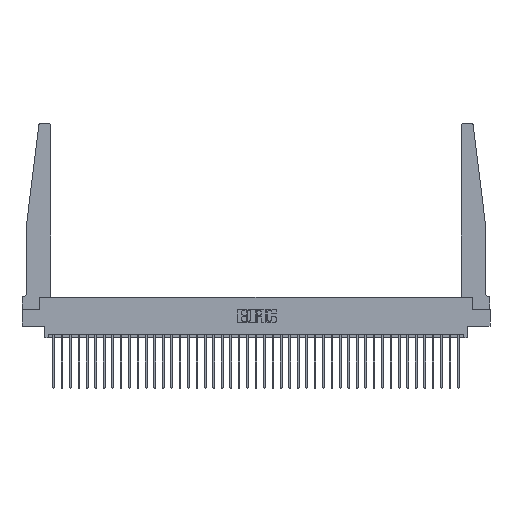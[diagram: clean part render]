
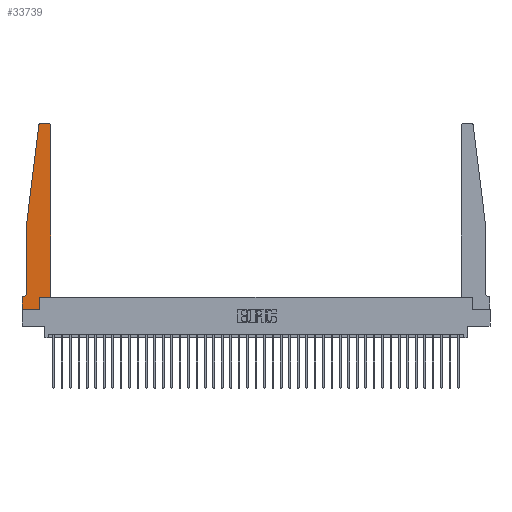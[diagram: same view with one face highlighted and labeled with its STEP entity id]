
A CAD part, top view. The second image highlights one B-rep face of the part: STEP entity #33739.
In plain terms, the highlighted planar face has unit normal (0, 0, 1).
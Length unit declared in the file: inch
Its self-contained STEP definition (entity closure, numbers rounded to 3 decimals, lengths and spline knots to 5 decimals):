
#533 = LINE ( 'NONE', #15064, #18620 ) ;
#2015 = DIRECTION ( 'NONE',  ( 0., -1., 0. ) ) ;
#3182 = ORIENTED_EDGE ( 'NONE', *, *, #14814, .T. ) ;
#3722 = VERTEX_POINT ( 'NONE', #31703 ) ;
#3955 = ORIENTED_EDGE ( 'NONE', *, *, #27358, .T. ) ;
#4092 = CARTESIAN_POINT ( 'NONE',  ( 0.065, 1.25, 0.37 ) ) ;
#4121 = LINE ( 'NONE', #35596, #8197 ) ;
#4212 = DIRECTION ( 'NONE',  ( 0., 0., 1. ) ) ;
#5994 = VERTEX_POINT ( 'NONE', #32559 ) ;
#6804 = AXIS2_PLACEMENT_3D ( 'NONE', #6951, #4212, #15423 ) ;
#6951 = CARTESIAN_POINT ( 'NONE',  ( 0.27653, 2.72, 0.37 ) ) ;
#8189 = ORIENTED_EDGE ( 'NONE', *, *, #26859, .T. ) ;
#8197 = VECTOR ( 'NONE', #18302, 39.37008 ) ;
#8276 = DIRECTION ( 'NONE',  ( 1., 0., 0. ) ) ;
#8376 = DIRECTION ( 'NONE',  ( 0., 1., 0. ) ) ;
#8692 = ORIENTED_EDGE ( 'NONE', *, *, #8763, .T. ) ;
#8763 = EDGE_CURVE ( 'NONE', #23755, #24429, #22695, .T. ) ;
#10007 = ORIENTED_EDGE ( 'NONE', *, *, #18033, .T. ) ;
#10008 = LINE ( 'NONE', #12965, #21346 ) ;
#10170 = LINE ( 'NONE', #32835, #20665 ) ;
#10447 = EDGE_CURVE ( 'NONE', #18459, #13462, #26525, .T. ) ;
#10569 = EDGE_CURVE ( 'NONE', #24429, #34823, #533, .T. ) ;
#11176 = CIRCLE ( 'NONE', #24096, 0.05 ) ;
#11351 = EDGE_CURVE ( 'NONE', #5994, #3722, #34732, .T. ) ;
#11415 = CARTESIAN_POINT ( 'NONE',  ( 0.395, 2.72, 0.37 ) ) ;
#11577 = VERTEX_POINT ( 'NONE', #29917 ) ;
#11580 = AXIS2_PLACEMENT_3D ( 'NONE', #13232, #24849, #8276 ) ;
#11585 = EDGE_CURVE ( 'NONE', #26230, #23755, #32330, .T. ) ;
#11857 = ORIENTED_EDGE ( 'NONE', *, *, #11585, .T. ) ;
#12165 = CARTESIAN_POINT ( 'NONE',  ( 0.27653, 2.75, 0.37 ) ) ;
#12965 = CARTESIAN_POINT ( 'NONE',  ( 0.425, 0.18, 0.37 ) ) ;
#13069 = FACE_OUTER_BOUND ( 'NONE', #33677, .T. ) ;
#13232 = CARTESIAN_POINT ( 'NONE',  ( 0., 0.1875, 0.37 ) ) ;
#13240 = CARTESIAN_POINT ( 'NONE',  ( 0.425, 2.72, 0.37 ) ) ;
#13246 = CARTESIAN_POINT ( 'NONE',  ( 0., 0., 0.37 ) ) ;
#13462 = VERTEX_POINT ( 'NONE', #34271 ) ;
#13972 = VECTOR ( 'NONE', #34342, 39.37008 ) ;
#14007 = VERTEX_POINT ( 'NONE', #13240 ) ;
#14814 = EDGE_CURVE ( 'NONE', #31611, #14007, #4121, .T. ) ;
#15064 = CARTESIAN_POINT ( 'NONE',  ( 0.065, 1.25, 0.37 ) ) ;
#15070 = AXIS2_PLACEMENT_3D ( 'NONE', #11415, #36309, #22477 ) ;
#15195 = ORIENTED_EDGE ( 'NONE', *, *, #30881, .T. ) ;
#15366 = CARTESIAN_POINT ( 'NONE',  ( 0.25, 2.75, 0.37 ) ) ;
#15423 = DIRECTION ( 'NONE',  ( 1., 0., 0. ) ) ;
#15763 = CARTESIAN_POINT ( 'NONE',  ( 0.395, 2.75, 0.37 ) ) ;
#15813 = VERTEX_POINT ( 'NONE', #19646 ) ;
#16169 = DIRECTION ( 'NONE',  ( -1., 0., 0. ) ) ;
#17201 = ORIENTED_EDGE ( 'NONE', *, *, #28276, .T. ) ;
#17674 = CARTESIAN_POINT ( 'NONE',  ( 0.065, 0.1875, 0.37 ) ) ;
#17844 = DIRECTION ( 'NONE',  ( -1., 0., 0. ) ) ;
#18033 = EDGE_CURVE ( 'NONE', #3722, #11577, #22374, .T. ) ;
#18302 = DIRECTION ( 'NONE',  ( 0., 1., 0. ) ) ;
#18459 = VERTEX_POINT ( 'NONE', #34451 ) ;
#18563 = DIRECTION ( 'NONE',  ( 0., 0., -1. ) ) ;
#18593 = LINE ( 'NONE', #13246, #29553 ) ;
#18620 = VECTOR ( 'NONE', #26312, 39.37008 ) ;
#19646 = CARTESIAN_POINT ( 'NONE',  ( 0.065, 0.2375, 0.37 ) ) ;
#19759 = ORIENTED_EDGE ( 'NONE', *, *, #10447, .T. ) ;
#20665 = VECTOR ( 'NONE', #21403, 39.37008 ) ;
#21237 = DIRECTION ( 'NONE',  ( 1., 0., 0. ) ) ;
#21346 = VECTOR ( 'NONE', #21237, 39.37008 ) ;
#21403 = DIRECTION ( 'NONE',  ( 0., -1., 0. ) ) ;
#22374 = LINE ( 'NONE', #33625, #22759 ) ;
#22477 = DIRECTION ( 'NONE',  ( 1., 0., 0. ) ) ;
#22695 = CIRCLE ( 'NONE', #6804, 0.03 ) ;
#22737 = CARTESIAN_POINT ( 'NONE',  ( 0., 0., 0.37 ) ) ;
#22759 = VECTOR ( 'NONE', #8376, 39.37008 ) ;
#23294 = CIRCLE ( 'NONE', #15070, 0.03 ) ;
#23731 = CARTESIAN_POINT ( 'NONE',  ( 0.015, 0.2375, 0.37 ) ) ;
#23755 = VERTEX_POINT ( 'NONE', #12165 ) ;
#23822 = DIRECTION ( 'NONE',  ( -1., 0., 0. ) ) ;
#24096 = AXIS2_PLACEMENT_3D ( 'NONE', #23731, #18563, #16169 ) ;
#24198 = ORIENTED_EDGE ( 'NONE', *, *, #10569, .T. ) ;
#24429 = VERTEX_POINT ( 'NONE', #26687 ) ;
#24464 = EDGE_CURVE ( 'NONE', #15813, #18459, #11176, .T. ) ;
#24669 = PLANE ( 'NONE',  #11580 ) ;
#24849 = DIRECTION ( 'NONE',  ( 0., 0., 1. ) ) ;
#25826 = CARTESIAN_POINT ( 'NONE',  ( 0.425, 0.18, 0.37 ) ) ;
#26230 = VERTEX_POINT ( 'NONE', #15763 ) ;
#26312 = DIRECTION ( 'NONE',  ( -0.122, -0.992, 0. ) ) ;
#26525 = LINE ( 'NONE', #17674, #33365 ) ;
#26687 = CARTESIAN_POINT ( 'NONE',  ( 0.24675, 2.72367, 0.37 ) ) ;
#26859 = EDGE_CURVE ( 'NONE', #34823, #15813, #10170, .T. ) ;
#27358 = EDGE_CURVE ( 'NONE', #13462, #5994, #18593, .T. ) ;
#28276 = EDGE_CURVE ( 'NONE', #11577, #31611, #10008, .T. ) ;
#29553 = VECTOR ( 'NONE', #2015, 39.37008 ) ;
#29917 = CARTESIAN_POINT ( 'NONE',  ( 0.2605, 0.18, 0.37 ) ) ;
#30881 = EDGE_CURVE ( 'NONE', #14007, #26230, #23294, .T. ) ;
#31611 = VERTEX_POINT ( 'NONE', #25826 ) ;
#31703 = CARTESIAN_POINT ( 'NONE',  ( 0.2605, 0., 0.37 ) ) ;
#32141 = ORIENTED_EDGE ( 'NONE', *, *, #11351, .T. ) ;
#32330 = LINE ( 'NONE', #15366, #32809 ) ;
#32559 = CARTESIAN_POINT ( 'NONE',  ( 0., 0., 0.37 ) ) ;
#32809 = VECTOR ( 'NONE', #23822, 39.37008 ) ;
#32835 = CARTESIAN_POINT ( 'NONE',  ( 0.065, 1.25, 0.37 ) ) ;
#33365 = VECTOR ( 'NONE', #17844, 39.37008 ) ;
#33625 = CARTESIAN_POINT ( 'NONE',  ( 0.2605, 0.18, 0.37 ) ) ;
#33677 = EDGE_LOOP ( 'NONE', ( #11857, #8692, #24198, #8189, #35992, #19759, #3955, #32141, #10007, #17201, #3182, #15195 ) ) ;
#33739 = ADVANCED_FACE ( 'NONE', ( #13069 ), #24669, .T. ) ;
#34271 = CARTESIAN_POINT ( 'NONE',  ( 0., 0.1875, 0.37 ) ) ;
#34342 = DIRECTION ( 'NONE',  ( 1., 0., 0. ) ) ;
#34451 = CARTESIAN_POINT ( 'NONE',  ( 0.015, 0.1875, 0.37 ) ) ;
#34732 = LINE ( 'NONE', #22737, #13972 ) ;
#34823 = VERTEX_POINT ( 'NONE', #4092 ) ;
#35596 = CARTESIAN_POINT ( 'NONE',  ( 0.425, 0.18, 0.37 ) ) ;
#35992 = ORIENTED_EDGE ( 'NONE', *, *, #24464, .T. ) ;
#36309 = DIRECTION ( 'NONE',  ( 0., 0., 1. ) ) ;
